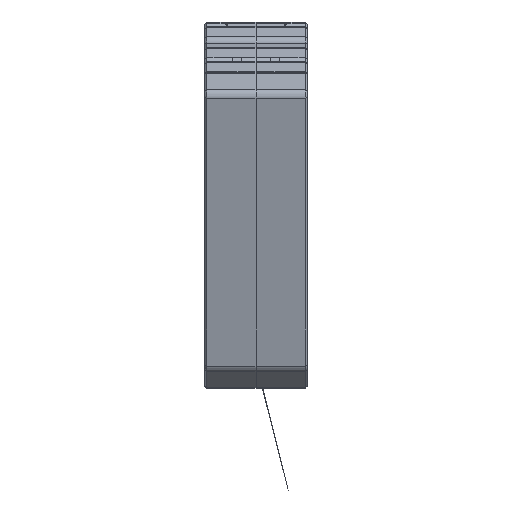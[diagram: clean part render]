
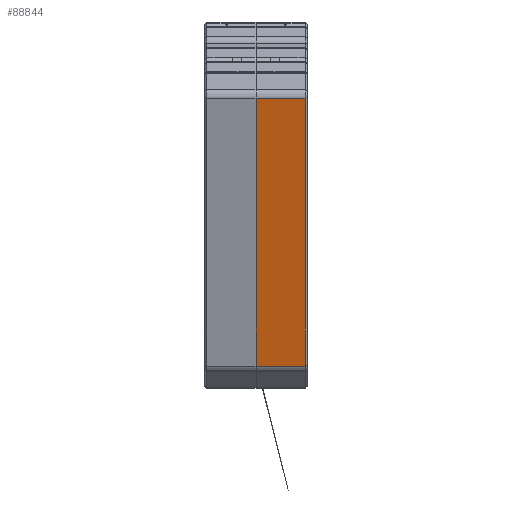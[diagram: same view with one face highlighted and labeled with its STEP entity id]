
A CAD part, front view. The second image highlights one B-rep face of the part: STEP entity #88844.
In plain terms, the highlighted planar face has unit normal (0, -0.97, -0.241).
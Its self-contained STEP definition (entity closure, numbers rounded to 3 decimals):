
#3781 = DIRECTION ( 'NONE',  ( -1., 0., 0. ) ) ;
#4228 = LINE ( 'NONE', #5384, #14463 ) ;
#5384 = CARTESIAN_POINT ( 'NONE',  ( 79.551, -101.021, -43.469 ) ) ;
#9759 = CARTESIAN_POINT ( 'NONE',  ( 12.252, -101.021, -43.469 ) ) ;
#11205 = VERTEX_POINT ( 'NONE', #9759 ) ;
#14463 = VECTOR ( 'NONE', #76612, 1000. ) ;
#15712 = DIRECTION ( 'NONE',  ( 0., -0.97, -0.241 ) ) ;
#21453 = CARTESIAN_POINT ( 'NONE',  ( 12.252, -105.317, -26.203 ) ) ;
#24601 = ORIENTED_EDGE ( 'NONE', *, *, #69467, .F. ) ;
#26774 = EDGE_CURVE ( 'NONE', #11205, #89824, #86049, .T. ) ;
#34843 = FACE_OUTER_BOUND ( 'NONE', #45457, .T. ) ;
#35673 = AXIS2_PLACEMENT_3D ( 'NONE', #107208, #15712, #79128 ) ;
#38246 = DIRECTION ( 'NONE',  ( 0., -0.241, 0.97 ) ) ;
#39034 = VECTOR ( 'NONE', #3781, 1000. ) ;
#39850 = VECTOR ( 'NONE', #38246, 1000. ) ;
#41888 = ORIENTED_EDGE ( 'NONE', *, *, #94544, .T. ) ;
#45457 = EDGE_LOOP ( 'NONE', ( #88710, #109034, #41888, #24601 ) ) ;
#45763 = EDGE_CURVE ( 'NONE', #88161, #11205, #4228, .T. ) ;
#49569 = CARTESIAN_POINT ( 'NONE',  ( 12.252, -117.611, 23.208 ) ) ;
#62981 = PLANE ( 'NONE',  #35673 ) ;
#69467 = EDGE_CURVE ( 'NONE', #88161, #115655, #69901, .T. ) ;
#69901 = LINE ( 'NONE', #97971, #92055 ) ;
#76612 = DIRECTION ( 'NONE',  ( 1., 0., 0. ) ) ;
#79128 = DIRECTION ( 'NONE',  ( 0., 0.241, -0.97 ) ) ;
#80942 = CARTESIAN_POINT ( 'NONE',  ( 0., -101.021, -43.469 ) ) ;
#85677 = CARTESIAN_POINT ( 'NONE',  ( 35.962, -117.611, 23.208 ) ) ;
#86049 = LINE ( 'NONE', #21453, #39850 ) ;
#87814 = DIRECTION ( 'NONE',  ( 0., -0.241, 0.97 ) ) ;
#88161 = VERTEX_POINT ( 'NONE', #80942 ) ;
#88710 = ORIENTED_EDGE ( 'NONE', *, *, #45763, .T. ) ;
#88844 = ADVANCED_FACE ( 'NONE', ( #34843 ), #62981, .T. ) ;
#89824 = VERTEX_POINT ( 'NONE', #49569 ) ;
#92055 = VECTOR ( 'NONE', #87814, 1000. ) ;
#94544 = EDGE_CURVE ( 'NONE', #89824, #115655, #106567, .T. ) ;
#97669 = CARTESIAN_POINT ( 'NONE',  ( 0., -117.611, 23.208 ) ) ;
#97971 = CARTESIAN_POINT ( 'NONE',  ( 0., -105.317, -26.203 ) ) ;
#106567 = LINE ( 'NONE', #85677, #39034 ) ;
#107208 = CARTESIAN_POINT ( 'NONE',  ( 79.551, -105.317, -26.203 ) ) ;
#109034 = ORIENTED_EDGE ( 'NONE', *, *, #26774, .T. ) ;
#115655 = VERTEX_POINT ( 'NONE', #97669 ) ;
